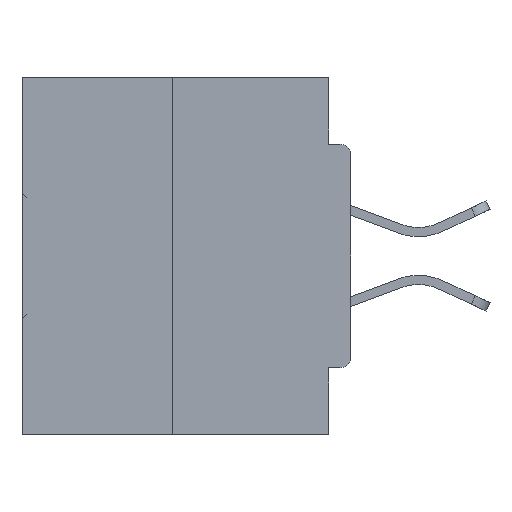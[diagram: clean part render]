
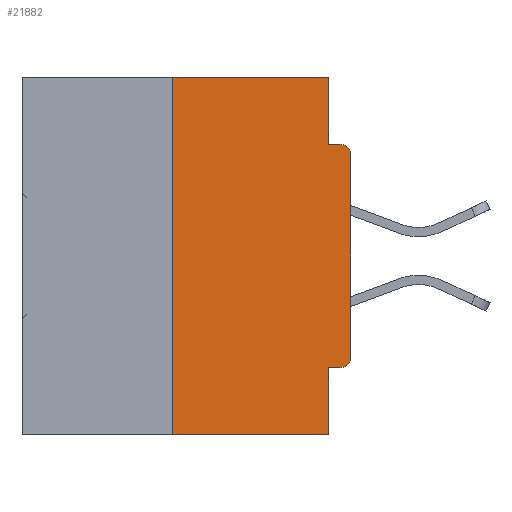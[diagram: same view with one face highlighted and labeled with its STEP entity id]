
A CAD part, left-side view. The second image highlights one B-rep face of the part: STEP entity #21882.
In plain terms, the highlighted planar face has unit normal (-1, 0, 0).
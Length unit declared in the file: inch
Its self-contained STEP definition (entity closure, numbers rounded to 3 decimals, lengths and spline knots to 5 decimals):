
#1042 = ORIENTED_EDGE ( 'NONE', *, *, #7074, .F. ) ;
#1254 = AXIS2_PLACEMENT_3D ( 'NONE', #21966, #39566, #22187 ) ;
#1345 = DIRECTION ( 'NONE',  ( 0., 0., -1. ) ) ;
#1788 = CARTESIAN_POINT ( 'NONE',  ( 0., 0.015, -0.3915 ) ) ;
#3100 = CARTESIAN_POINT ( 'NONE',  ( 0., 0., -0.3915 ) ) ;
#3170 = VERTEX_POINT ( 'NONE', #13977 ) ;
#3278 = VERTEX_POINT ( 'NONE', #38880 ) ;
#4023 = CARTESIAN_POINT ( 'NONE',  ( 0., 0.031, 0. ) ) ;
#4237 = EDGE_CURVE ( 'NONE', #3278, #39994, #40603, .T. ) ;
#4437 = ORIENTED_EDGE ( 'NONE', *, *, #10012, .F. ) ;
#4995 = DIRECTION ( 'NONE',  ( -1., 0., 0. ) ) ;
#5657 = CARTESIAN_POINT ( 'NONE',  ( 0., 0., -0.4065 ) ) ;
#7074 = EDGE_CURVE ( 'NONE', #13530, #27120, #8353, .T. ) ;
#7556 = LINE ( 'NONE', #21963, #12918 ) ;
#8070 = CARTESIAN_POINT ( 'NONE',  ( 0., 0.46, 0. ) ) ;
#8203 = EDGE_CURVE ( 'NONE', #30554, #27120, #20927, .T. ) ;
#8353 = LINE ( 'NONE', #29385, #26702 ) ;
#8997 = CARTESIAN_POINT ( 'NONE',  ( 0., 0.031, 0. ) ) ;
#9252 = DIRECTION ( 'NONE',  ( 0., -1., 0. ) ) ;
#9452 = DIRECTION ( 'NONE',  ( 0., -1., 0. ) ) ;
#9536 = EDGE_CURVE ( 'NONE', #42059, #30554, #37036, .T. ) ;
#9576 = CARTESIAN_POINT ( 'NONE',  ( 0., 0., 0. ) ) ;
#10012 = EDGE_CURVE ( 'NONE', #29940, #13530, #40728, .T. ) ;
#12578 = DIRECTION ( 'NONE',  ( 0., 0., 1. ) ) ;
#12809 = ORIENTED_EDGE ( 'NONE', *, *, #8203, .T. ) ;
#12864 = CIRCLE ( 'NONE', #44270, 0.015 ) ;
#12918 = VECTOR ( 'NONE', #15720, 39.37008 ) ;
#13055 = CARTESIAN_POINT ( 'NONE',  ( 0., 0.031, -0.0935 ) ) ;
#13530 = VERTEX_POINT ( 'NONE', #13055 ) ;
#13977 = CARTESIAN_POINT ( 'NONE',  ( 0., 0.031, -0.5 ) ) ;
#14301 = EDGE_CURVE ( 'NONE', #38805, #3170, #38481, .T. ) ;
#14857 = EDGE_CURVE ( 'NONE', #39994, #3170, #7556, .T. ) ;
#15720 = DIRECTION ( 'NONE',  ( 0., 0., -1. ) ) ;
#15831 = DIRECTION ( 'NONE',  ( 0., 0., 1. ) ) ;
#16116 = CARTESIAN_POINT ( 'NONE',  ( 0., 0.25, 0. ) ) ;
#16859 = VECTOR ( 'NONE', #12578, 39.37008 ) ;
#17918 = ORIENTED_EDGE ( 'NONE', *, *, #14857, .F. ) ;
#18428 = ORIENTED_EDGE ( 'NONE', *, *, #29627, .T. ) ;
#19464 = ORIENTED_EDGE ( 'NONE', *, *, #14301, .T. ) ;
#19572 = VECTOR ( 'NONE', #31631, 39.37008 ) ;
#19942 = DIRECTION ( 'NONE',  ( 0., 0., -1. ) ) ;
#20067 = VERTEX_POINT ( 'NONE', #16116 ) ;
#20927 = CIRCLE ( 'NONE', #1254, 0.015 ) ;
#21519 = ORIENTED_EDGE ( 'NONE', *, *, #4237, .F. ) ;
#21882 = ADVANCED_FACE ( 'NONE', ( #25637 ), #22659, .F. ) ;
#21963 = CARTESIAN_POINT ( 'NONE',  ( 0., 0.031, -0.5 ) ) ;
#21966 = CARTESIAN_POINT ( 'NONE',  ( 0., 0.015, -0.1085 ) ) ;
#22004 = DIRECTION ( 'NONE',  ( 0., 0., -1. ) ) ;
#22162 = CARTESIAN_POINT ( 'NONE',  ( 0., 0.031, -0.4065 ) ) ;
#22187 = DIRECTION ( 'NONE',  ( 0., 0., -1. ) ) ;
#22471 = ORIENTED_EDGE ( 'NONE', *, *, #28672, .F. ) ;
#22659 = PLANE ( 'NONE',  #32941 ) ;
#23101 = EDGE_LOOP ( 'NONE', ( #39320, #22471, #19464, #17918, #21519, #18428, #38122, #12809, #1042, #4437 ) ) ;
#23130 = LINE ( 'NONE', #36424, #42768 ) ;
#25637 = FACE_OUTER_BOUND ( 'NONE', #23101, .T. ) ;
#26595 = VECTOR ( 'NONE', #27100, 39.37008 ) ;
#26702 = VECTOR ( 'NONE', #9452, 39.37008 ) ;
#27100 = DIRECTION ( 'NONE',  ( 0., 1., 0. ) ) ;
#27120 = VERTEX_POINT ( 'NONE', #40996 ) ;
#28489 = LINE ( 'NONE', #42417, #40681 ) ;
#28672 = EDGE_CURVE ( 'NONE', #38805, #20067, #23130, .T. ) ;
#29385 = CARTESIAN_POINT ( 'NONE',  ( 0., 0., -0.0935 ) ) ;
#29627 = EDGE_CURVE ( 'NONE', #3278, #42059, #12864, .T. ) ;
#29940 = VERTEX_POINT ( 'NONE', #4023 ) ;
#30554 = VERTEX_POINT ( 'NONE', #39831 ) ;
#31530 = VECTOR ( 'NONE', #19942, 39.37008 ) ;
#31631 = DIRECTION ( 'NONE',  ( 0., -1., 0. ) ) ;
#32941 = AXIS2_PLACEMENT_3D ( 'NONE', #8070, #43036, #22004 ) ;
#36424 = CARTESIAN_POINT ( 'NONE',  ( 0., 0.25, 0. ) ) ;
#37036 = LINE ( 'NONE', #9576, #16859 ) ;
#38015 = CARTESIAN_POINT ( 'NONE',  ( 0., 0.46, -0.5 ) ) ;
#38122 = ORIENTED_EDGE ( 'NONE', *, *, #9536, .T. ) ;
#38481 = LINE ( 'NONE', #38015, #19572 ) ;
#38805 = VERTEX_POINT ( 'NONE', #40195 ) ;
#38880 = CARTESIAN_POINT ( 'NONE',  ( 0., 0.015, -0.4065 ) ) ;
#39320 = ORIENTED_EDGE ( 'NONE', *, *, #40887, .F. ) ;
#39566 = DIRECTION ( 'NONE',  ( -1., 0., 0. ) ) ;
#39831 = CARTESIAN_POINT ( 'NONE',  ( 0., 0., -0.1085 ) ) ;
#39994 = VERTEX_POINT ( 'NONE', #22162 ) ;
#40195 = CARTESIAN_POINT ( 'NONE',  ( 0., 0.25, -0.5 ) ) ;
#40603 = LINE ( 'NONE', #5657, #26595 ) ;
#40681 = VECTOR ( 'NONE', #9252, 39.37008 ) ;
#40728 = LINE ( 'NONE', #8997, #31530 ) ;
#40887 = EDGE_CURVE ( 'NONE', #20067, #29940, #28489, .T. ) ;
#40996 = CARTESIAN_POINT ( 'NONE',  ( 0., 0.015, -0.0935 ) ) ;
#42059 = VERTEX_POINT ( 'NONE', #3100 ) ;
#42417 = CARTESIAN_POINT ( 'NONE',  ( 0., 0.46, 0. ) ) ;
#42768 = VECTOR ( 'NONE', #15831, 39.37008 ) ;
#43036 = DIRECTION ( 'NONE',  ( 1., 0., 0. ) ) ;
#44270 = AXIS2_PLACEMENT_3D ( 'NONE', #1788, #4995, #1345 ) ;
